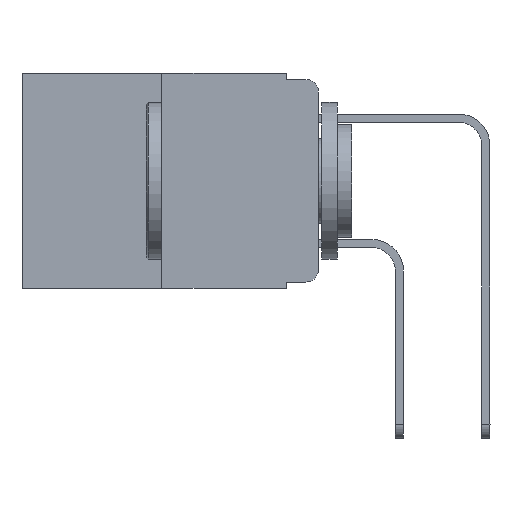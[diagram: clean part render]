
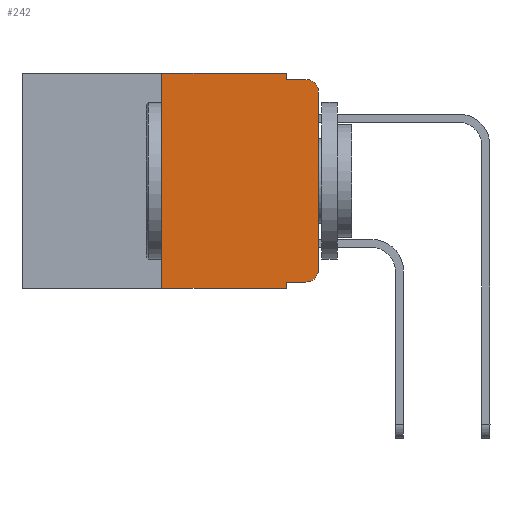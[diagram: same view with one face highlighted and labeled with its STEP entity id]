
A CAD part, left-side view. The second image highlights one B-rep face of the part: STEP entity #242.
In plain terms, the highlighted planar face has unit normal (-1, 0, 0).
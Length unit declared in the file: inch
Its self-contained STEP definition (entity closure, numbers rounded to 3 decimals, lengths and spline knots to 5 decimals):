
#3 = CARTESIAN_POINT ( 'NONE',  ( 0., 0.473, 0. ) ) ;
#70 = LINE ( 'NONE', #2944, #10407 ) ;
#92 = ORIENTED_EDGE ( 'NONE', *, *, #4015, .T. ) ;
#128 = DIRECTION ( 'NONE',  ( 0., -1., 0. ) ) ;
#173 = CIRCLE ( 'NONE', #5751, 0.02 ) ;
#242 = ADVANCED_FACE ( 'NONE', ( #11230 ), #854, .F. ) ;
#468 = VERTEX_POINT ( 'NONE', #11831 ) ;
#854 = PLANE ( 'NONE',  #2905 ) ;
#977 = ORIENTED_EDGE ( 'NONE', *, *, #5894, .F. ) ;
#1392 = CARTESIAN_POINT ( 'NONE',  ( 0., 0.02, -0.01 ) ) ;
#1585 = CARTESIAN_POINT ( 'NONE',  ( 0., 0., 0. ) ) ;
#1664 = EDGE_CURVE ( 'NONE', #11420, #10656, #5943, .T. ) ;
#1699 = VERTEX_POINT ( 'NONE', #10464 ) ;
#1778 = DIRECTION ( 'NONE',  ( 0., 0., -1. ) ) ;
#1974 = CARTESIAN_POINT ( 'NONE',  ( 0., 0., -0.313 ) ) ;
#2059 = VERTEX_POINT ( 'NONE', #9515 ) ;
#2118 = CARTESIAN_POINT ( 'NONE',  ( 0., 0.473, -0.343 ) ) ;
#2125 = ORIENTED_EDGE ( 'NONE', *, *, #8133, .T. ) ;
#2414 = DIRECTION ( 'NONE',  ( 0., 0., -1. ) ) ;
#2496 = DIRECTION ( 'NONE',  ( 0., -1., 0. ) ) ;
#2499 = CARTESIAN_POINT ( 'NONE',  ( 0., 0.02, -0.03 ) ) ;
#2502 = VECTOR ( 'NONE', #2414, 39.37008 ) ;
#2542 = VERTEX_POINT ( 'NONE', #10791 ) ;
#2905 = AXIS2_PLACEMENT_3D ( 'NONE', #4643, #4515, #6375 ) ;
#2944 = CARTESIAN_POINT ( 'NONE',  ( 0., 0.25, 0. ) ) ;
#3124 = EDGE_CURVE ( 'NONE', #7951, #2542, #6117, .T. ) ;
#3135 = DIRECTION ( 'NONE',  ( 0., -1., 0. ) ) ;
#3153 = ORIENTED_EDGE ( 'NONE', *, *, #11481, .F. ) ;
#3268 = AXIS2_PLACEMENT_3D ( 'NONE', #3649, #10187, #8234 ) ;
#3407 = LINE ( 'NONE', #11799, #2502 ) ;
#3414 = EDGE_CURVE ( 'NONE', #468, #4602, #70, .T. ) ;
#3649 = CARTESIAN_POINT ( 'NONE',  ( 0., 0.02, -0.313 ) ) ;
#3857 = LINE ( 'NONE', #2118, #6590 ) ;
#4015 = EDGE_CURVE ( 'NONE', #10656, #7951, #7224, .T. ) ;
#4117 = CARTESIAN_POINT ( 'NONE',  ( 0., 0.25, 0. ) ) ;
#4130 = CARTESIAN_POINT ( 'NONE',  ( 0., 0.051, -0.333 ) ) ;
#4162 = ORIENTED_EDGE ( 'NONE', *, *, #7004, .F. ) ;
#4436 = DIRECTION ( 'NONE',  ( 0., 0., 1. ) ) ;
#4459 = VERTEX_POINT ( 'NONE', #4632 ) ;
#4461 = LINE ( 'NONE', #11796, #9486 ) ;
#4515 = DIRECTION ( 'NONE',  ( 1., 0., 0. ) ) ;
#4602 = VERTEX_POINT ( 'NONE', #4117 ) ;
#4632 = CARTESIAN_POINT ( 'NONE',  ( 0., 0.051, -0.01 ) ) ;
#4643 = CARTESIAN_POINT ( 'NONE',  ( 0., 0.473, 0. ) ) ;
#5380 = VECTOR ( 'NONE', #3135, 39.37008 ) ;
#5649 = ORIENTED_EDGE ( 'NONE', *, *, #3124, .T. ) ;
#5751 = AXIS2_PLACEMENT_3D ( 'NONE', #2499, #12078, #1778 ) ;
#5894 = EDGE_CURVE ( 'NONE', #11420, #1699, #3407, .T. ) ;
#5943 = LINE ( 'NONE', #9589, #5380 ) ;
#6063 = ORIENTED_EDGE ( 'NONE', *, *, #1664, .T. ) ;
#6117 = LINE ( 'NONE', #1585, #7804 ) ;
#6375 = DIRECTION ( 'NONE',  ( 0., 0., -1. ) ) ;
#6530 = CARTESIAN_POINT ( 'NONE',  ( 0., 0.02, -0.333 ) ) ;
#6590 = VECTOR ( 'NONE', #7631, 39.37008 ) ;
#6737 = DIRECTION ( 'NONE',  ( 0., 0., 1. ) ) ;
#7004 = EDGE_CURVE ( 'NONE', #4602, #2059, #11524, .T. ) ;
#7121 = DIRECTION ( 'NONE',  ( 0., 0., -1. ) ) ;
#7192 = EDGE_LOOP ( 'NONE', ( #5649, #2125, #3153, #11987, #4162, #11368, #10755, #977, #6063, #92 ) ) ;
#7216 = LINE ( 'NONE', #11018, #9124 ) ;
#7224 = CIRCLE ( 'NONE', #3268, 0.02 ) ;
#7631 = DIRECTION ( 'NONE',  ( 0., -1., 0. ) ) ;
#7804 = VECTOR ( 'NONE', #4436, 39.37008 ) ;
#7951 = VERTEX_POINT ( 'NONE', #1974 ) ;
#8133 = EDGE_CURVE ( 'NONE', #2542, #10172, #173, .T. ) ;
#8234 = DIRECTION ( 'NONE',  ( 0., 0., -1. ) ) ;
#9124 = VECTOR ( 'NONE', #2496, 39.37008 ) ;
#9235 = EDGE_CURVE ( 'NONE', #2059, #4459, #4461, .T. ) ;
#9486 = VECTOR ( 'NONE', #7121, 39.37008 ) ;
#9515 = CARTESIAN_POINT ( 'NONE',  ( 0., 0.051, 0. ) ) ;
#9589 = CARTESIAN_POINT ( 'NONE',  ( 0., 0.051, -0.333 ) ) ;
#10172 = VERTEX_POINT ( 'NONE', #1392 ) ;
#10187 = DIRECTION ( 'NONE',  ( -1., 0., 0. ) ) ;
#10407 = VECTOR ( 'NONE', #6737, 39.37008 ) ;
#10464 = CARTESIAN_POINT ( 'NONE',  ( 0., 0.051, -0.343 ) ) ;
#10656 = VERTEX_POINT ( 'NONE', #6530 ) ;
#10755 = ORIENTED_EDGE ( 'NONE', *, *, #12174, .T. ) ;
#10791 = CARTESIAN_POINT ( 'NONE',  ( 0., 0., -0.03 ) ) ;
#11018 = CARTESIAN_POINT ( 'NONE',  ( 0., 0.051, -0.01 ) ) ;
#11230 = FACE_OUTER_BOUND ( 'NONE', #7192, .T. ) ;
#11368 = ORIENTED_EDGE ( 'NONE', *, *, #3414, .F. ) ;
#11420 = VERTEX_POINT ( 'NONE', #4130 ) ;
#11481 = EDGE_CURVE ( 'NONE', #4459, #10172, #7216, .T. ) ;
#11524 = LINE ( 'NONE', #3, #12053 ) ;
#11796 = CARTESIAN_POINT ( 'NONE',  ( 0., 0.051, 0. ) ) ;
#11799 = CARTESIAN_POINT ( 'NONE',  ( 0., 0.051, 0. ) ) ;
#11831 = CARTESIAN_POINT ( 'NONE',  ( 0., 0.25, -0.343 ) ) ;
#11987 = ORIENTED_EDGE ( 'NONE', *, *, #9235, .F. ) ;
#12053 = VECTOR ( 'NONE', #128, 39.37008 ) ;
#12078 = DIRECTION ( 'NONE',  ( -1., 0., 0. ) ) ;
#12174 = EDGE_CURVE ( 'NONE', #468, #1699, #3857, .T. ) ;
